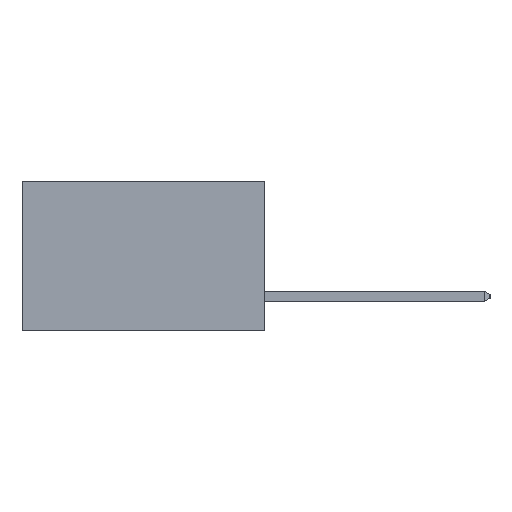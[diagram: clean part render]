
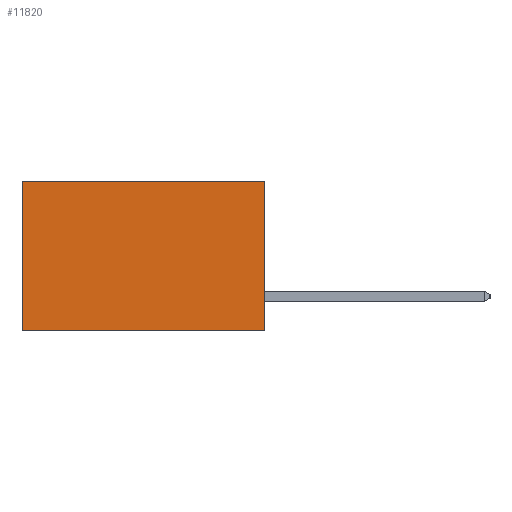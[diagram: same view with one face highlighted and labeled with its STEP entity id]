
A CAD part, left-side view. The second image highlights one B-rep face of the part: STEP entity #11820.
In plain terms, the highlighted planar face has unit normal (-1, 0, 0).
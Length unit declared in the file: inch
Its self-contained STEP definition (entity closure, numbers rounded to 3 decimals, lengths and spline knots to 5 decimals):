
#39 = CARTESIAN_POINT ( 'NONE',  ( 0.2615, 0.6, -0.37 ) ) ;
#412 = ORIENTED_EDGE ( 'NONE', *, *, #488, .F. ) ;
#488 = EDGE_CURVE ( 'NONE', #9007, #9533, #13420, .T. ) ;
#673 = ORIENTED_EDGE ( 'NONE', *, *, #3112, .T. ) ;
#761 = DIRECTION ( 'NONE',  ( 0., 0., -1. ) ) ;
#981 = PLANE ( 'NONE',  #10811 ) ;
#1040 = LINE ( 'NONE', #9801, #7050 ) ;
#1237 = VERTEX_POINT ( 'NONE', #2436 ) ;
#1296 = FACE_OUTER_BOUND ( 'NONE', #6579, .T. ) ;
#2120 = DIRECTION ( 'NONE',  ( 0., 0., -1. ) ) ;
#2436 = CARTESIAN_POINT ( 'NONE',  ( 0.2615, 0.6, -0.37 ) ) ;
#2654 = CARTESIAN_POINT ( 'NONE',  ( 0.2615, 0., -0.37 ) ) ;
#3112 = EDGE_CURVE ( 'NONE', #9007, #6417, #1040, .T. ) ;
#3267 = DIRECTION ( 'NONE',  ( 0., 1., 0. ) ) ;
#3574 = CARTESIAN_POINT ( 'NONE',  ( 0.2615, 0., -0.37 ) ) ;
#4623 = DIRECTION ( 'NONE',  ( 0., 0., -1. ) ) ;
#4633 = VECTOR ( 'NONE', #761, 39.37008 ) ;
#5894 = CARTESIAN_POINT ( 'NONE',  ( 0.2615, 0.6, 0. ) ) ;
#6417 = VERTEX_POINT ( 'NONE', #5894 ) ;
#6579 = EDGE_LOOP ( 'NONE', ( #7855, #7848, #412, #673 ) ) ;
#6625 = CARTESIAN_POINT ( 'NONE',  ( 0.2615, 0., -0.37 ) ) ;
#6898 = VECTOR ( 'NONE', #3267, 39.37008 ) ;
#6958 = VECTOR ( 'NONE', #4623, 39.37008 ) ;
#7050 = VECTOR ( 'NONE', #9752, 39.37008 ) ;
#7848 = ORIENTED_EDGE ( 'NONE', *, *, #8052, .F. ) ;
#7855 = ORIENTED_EDGE ( 'NONE', *, *, #12434, .T. ) ;
#8052 = EDGE_CURVE ( 'NONE', #9533, #1237, #12428, .T. ) ;
#9007 = VERTEX_POINT ( 'NONE', #12671 ) ;
#9533 = VERTEX_POINT ( 'NONE', #3574 ) ;
#9752 = DIRECTION ( 'NONE',  ( 0., 1., 0. ) ) ;
#9801 = CARTESIAN_POINT ( 'NONE',  ( 0.2615, 0., 0. ) ) ;
#9984 = CARTESIAN_POINT ( 'NONE',  ( 0.2615, 0., -0.37 ) ) ;
#10811 = AXIS2_PLACEMENT_3D ( 'NONE', #6625, #13190, #2120 ) ;
#11820 = ADVANCED_FACE ( 'NONE', ( #1296 ), #981, .F. ) ;
#12428 = LINE ( 'NONE', #9984, #6898 ) ;
#12434 = EDGE_CURVE ( 'NONE', #6417, #1237, #12822, .T. ) ;
#12671 = CARTESIAN_POINT ( 'NONE',  ( 0.2615, 0., 0. ) ) ;
#12822 = LINE ( 'NONE', #39, #6958 ) ;
#13190 = DIRECTION ( 'NONE',  ( 1., 0., 0. ) ) ;
#13420 = LINE ( 'NONE', #2654, #4633 ) ;
